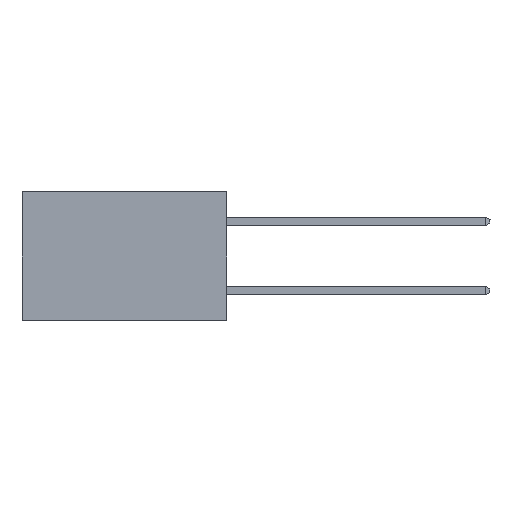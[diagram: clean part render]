
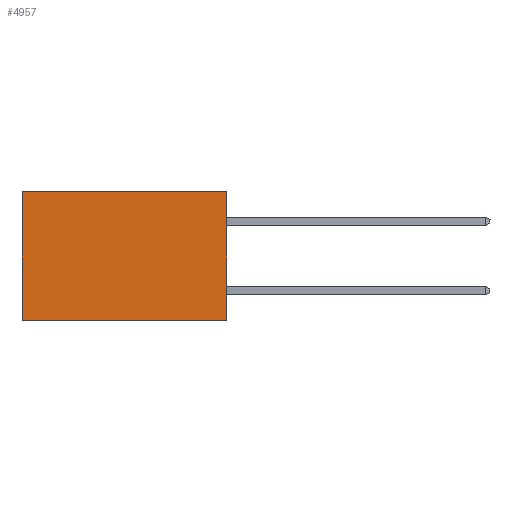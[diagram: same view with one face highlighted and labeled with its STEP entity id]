
A CAD part, left-side view. The second image highlights one B-rep face of the part: STEP entity #4957.
In plain terms, the highlighted planar face has unit normal (-1, 0, 0).
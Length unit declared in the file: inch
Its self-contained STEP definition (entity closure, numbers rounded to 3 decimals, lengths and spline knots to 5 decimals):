
#482 = DIRECTION ( 'NONE',  ( 0., 0., -1. ) ) ;
#546 = DIRECTION ( 'NONE',  ( 1., 0., 0. ) ) ;
#571 = CARTESIAN_POINT ( 'NONE',  ( 0.277, 0., -0.37 ) ) ;
#841 = PLANE ( 'NONE',  #15343 ) ;
#1714 = EDGE_LOOP ( 'NONE', ( #7437, #14736, #8953, #25173 ) ) ;
#1894 = VECTOR ( 'NONE', #13178, 39.37008 ) ;
#3673 = LINE ( 'NONE', #14128, #8605 ) ;
#3882 = VERTEX_POINT ( 'NONE', #11942 ) ;
#4957 = ADVANCED_FACE ( 'NONE', ( #21094 ), #841, .F. ) ;
#5113 = VERTEX_POINT ( 'NONE', #14566 ) ;
#5886 = CARTESIAN_POINT ( 'NONE',  ( 0.277, 0., 0. ) ) ;
#7437 = ORIENTED_EDGE ( 'NONE', *, *, #22536, .T. ) ;
#7868 = VECTOR ( 'NONE', #9093, 39.37008 ) ;
#8327 = EDGE_CURVE ( 'NONE', #3882, #13778, #13424, .T. ) ;
#8605 = VECTOR ( 'NONE', #24265, 39.37008 ) ;
#8953 = ORIENTED_EDGE ( 'NONE', *, *, #24188, .F. ) ;
#9093 = DIRECTION ( 'NONE',  ( 0., 1., 0. ) ) ;
#11047 = CARTESIAN_POINT ( 'NONE',  ( 0.277, 0., -0.37 ) ) ;
#11771 = VECTOR ( 'NONE', #12173, 39.37008 ) ;
#11942 = CARTESIAN_POINT ( 'NONE',  ( 0.277, 0., -0.37 ) ) ;
#12173 = DIRECTION ( 'NONE',  ( 0., 1., 0. ) ) ;
#13178 = DIRECTION ( 'NONE',  ( 0., 0., -1. ) ) ;
#13424 = LINE ( 'NONE', #21948, #7868 ) ;
#13778 = VERTEX_POINT ( 'NONE', #20637 ) ;
#14128 = CARTESIAN_POINT ( 'NONE',  ( 0.277, 0.59, -0.37 ) ) ;
#14566 = CARTESIAN_POINT ( 'NONE',  ( 0.277, 0., 0. ) ) ;
#14736 = ORIENTED_EDGE ( 'NONE', *, *, #8327, .F. ) ;
#15343 = AXIS2_PLACEMENT_3D ( 'NONE', #571, #546, #482 ) ;
#15961 = LINE ( 'NONE', #5886, #11771 ) ;
#16431 = CARTESIAN_POINT ( 'NONE',  ( 0.277, 0.59, 0. ) ) ;
#17804 = VERTEX_POINT ( 'NONE', #16431 ) ;
#18492 = LINE ( 'NONE', #11047, #1894 ) ;
#20637 = CARTESIAN_POINT ( 'NONE',  ( 0.277, 0.59, -0.37 ) ) ;
#21094 = FACE_OUTER_BOUND ( 'NONE', #1714, .T. ) ;
#21948 = CARTESIAN_POINT ( 'NONE',  ( 0.277, 0., -0.37 ) ) ;
#22536 = EDGE_CURVE ( 'NONE', #17804, #13778, #3673, .T. ) ;
#23854 = EDGE_CURVE ( 'NONE', #5113, #17804, #15961, .T. ) ;
#24188 = EDGE_CURVE ( 'NONE', #5113, #3882, #18492, .T. ) ;
#24265 = DIRECTION ( 'NONE',  ( 0., 0., -1. ) ) ;
#25173 = ORIENTED_EDGE ( 'NONE', *, *, #23854, .T. ) ;
